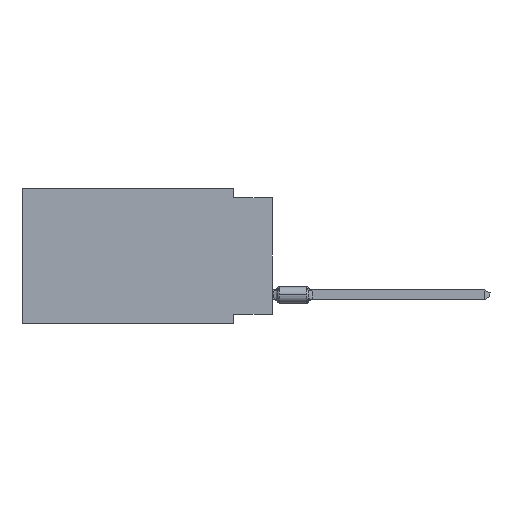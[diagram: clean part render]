
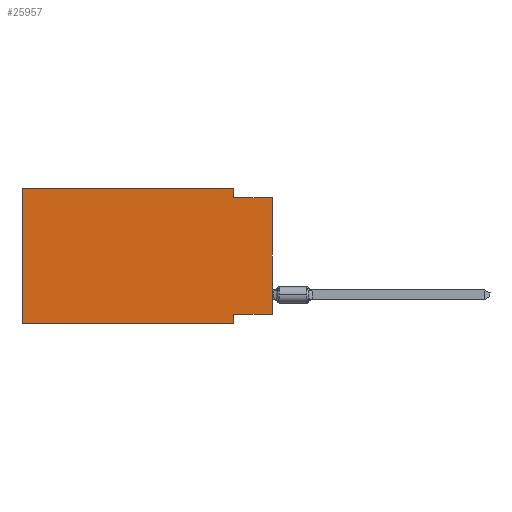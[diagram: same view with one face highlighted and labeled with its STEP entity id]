
A CAD part, left-side view. The second image highlights one B-rep face of the part: STEP entity #25957.
In plain terms, the highlighted planar face has unit normal (-1, 0, 0).
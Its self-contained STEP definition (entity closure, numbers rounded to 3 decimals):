
#1000 = DIRECTION ( 'NONE',  ( 0., 0., -1. ) ) ;
#1112 = DIRECTION ( 'NONE',  ( 0., 0., -1. ) ) ;
#1555 = ORIENTED_EDGE ( 'NONE', *, *, #27193, .F. ) ;
#2765 = ORIENTED_EDGE ( 'NONE', *, *, #39195, .F. ) ;
#4514 = CARTESIAN_POINT ( 'NONE',  ( 0., 2.54, 0. ) ) ;
#4989 = EDGE_CURVE ( 'NONE', #33740, #26155, #41452, .T. ) ;
#5279 = AXIS2_PLACEMENT_3D ( 'NONE', #33440, #35003, #1112 ) ;
#5985 = PLANE ( 'NONE',  #5279 ) ;
#6275 = LINE ( 'NONE', #20686, #9706 ) ;
#6925 = ORIENTED_EDGE ( 'NONE', *, *, #11265, .F. ) ;
#7074 = LINE ( 'NONE', #42701, #24734 ) ;
#8180 = FACE_OUTER_BOUND ( 'NONE', #15157, .T. ) ;
#8844 = LINE ( 'NONE', #19970, #28362 ) ;
#9148 = LINE ( 'NONE', #15763, #44595 ) ;
#9351 = ORIENTED_EDGE ( 'NONE', *, *, #15860, .F. ) ;
#9706 = VECTOR ( 'NONE', #35748, 1000. ) ;
#9810 = LINE ( 'NONE', #10257, #33088 ) ;
#10257 = CARTESIAN_POINT ( 'NONE',  ( 0., 16.383, 0. ) ) ;
#10415 = CARTESIAN_POINT ( 'NONE',  ( 0., 0., -8.255 ) ) ;
#11008 = CARTESIAN_POINT ( 'NONE',  ( 0., 16.383, 0. ) ) ;
#11265 = EDGE_CURVE ( 'NONE', #23553, #26155, #7074, .T. ) ;
#13021 = LINE ( 'NONE', #16814, #21232 ) ;
#13597 = CARTESIAN_POINT ( 'NONE',  ( 0., 0., 0. ) ) ;
#13998 = CARTESIAN_POINT ( 'NONE',  ( 0., 0., -0.635 ) ) ;
#15157 = EDGE_LOOP ( 'NONE', ( #38089, #6925, #9351, #1555, #43843, #21561, #2765, #21876 ) ) ;
#15763 = CARTESIAN_POINT ( 'NONE',  ( 0., 16.383, 0. ) ) ;
#15860 = EDGE_CURVE ( 'NONE', #34792, #23553, #33320, .T. ) ;
#16075 = CARTESIAN_POINT ( 'NONE',  ( 0., 2.54, -8.255 ) ) ;
#16814 = CARTESIAN_POINT ( 'NONE',  ( 0., 0., -8.255 ) ) ;
#19796 = DIRECTION ( 'NONE',  ( 0., -1., 0. ) ) ;
#19970 = CARTESIAN_POINT ( 'NONE',  ( 0., 16.383, -8.89 ) ) ;
#20492 = VERTEX_POINT ( 'NONE', #16075 ) ;
#20686 = CARTESIAN_POINT ( 'NONE',  ( 0., 2.54, -8.89 ) ) ;
#21076 = VECTOR ( 'NONE', #1000, 1000. ) ;
#21232 = VECTOR ( 'NONE', #38712, 1000. ) ;
#21561 = ORIENTED_EDGE ( 'NONE', *, *, #43914, .T. ) ;
#21876 = ORIENTED_EDGE ( 'NONE', *, *, #28725, .F. ) ;
#23553 = VERTEX_POINT ( 'NONE', #26669 ) ;
#24734 = VECTOR ( 'NONE', #35388, 1000. ) ;
#25062 = VECTOR ( 'NONE', #27729, 1000. ) ;
#25734 = VERTEX_POINT ( 'NONE', #45717 ) ;
#25957 = ADVANCED_FACE ( 'NONE', ( #8180 ), #5985, .F. ) ;
#26155 = VERTEX_POINT ( 'NONE', #13998 ) ;
#26669 = CARTESIAN_POINT ( 'NONE',  ( 0., 2.54, -0.635 ) ) ;
#26938 = VERTEX_POINT ( 'NONE', #46213 ) ;
#27193 = EDGE_CURVE ( 'NONE', #38830, #34792, #9148, .T. ) ;
#27729 = DIRECTION ( 'NONE',  ( 0., 0., 1. ) ) ;
#28362 = VECTOR ( 'NONE', #44728, 1000. ) ;
#28725 = EDGE_CURVE ( 'NONE', #33740, #20492, #13021, .T. ) ;
#33088 = VECTOR ( 'NONE', #42838, 1000. ) ;
#33320 = LINE ( 'NONE', #4514, #21076 ) ;
#33440 = CARTESIAN_POINT ( 'NONE',  ( 0., 16.383, 0. ) ) ;
#33740 = VERTEX_POINT ( 'NONE', #10415 ) ;
#34792 = VERTEX_POINT ( 'NONE', #34869 ) ;
#34869 = CARTESIAN_POINT ( 'NONE',  ( 0., 2.54, 0. ) ) ;
#35003 = DIRECTION ( 'NONE',  ( 1., 0., 0. ) ) ;
#35388 = DIRECTION ( 'NONE',  ( 0., -1., 0. ) ) ;
#35517 = EDGE_CURVE ( 'NONE', #26938, #38830, #9810, .T. ) ;
#35748 = DIRECTION ( 'NONE',  ( 0., 0., -1. ) ) ;
#38089 = ORIENTED_EDGE ( 'NONE', *, *, #4989, .T. ) ;
#38712 = DIRECTION ( 'NONE',  ( 0., 1., 0. ) ) ;
#38830 = VERTEX_POINT ( 'NONE', #11008 ) ;
#39195 = EDGE_CURVE ( 'NONE', #20492, #25734, #6275, .T. ) ;
#41452 = LINE ( 'NONE', #13597, #25062 ) ;
#42701 = CARTESIAN_POINT ( 'NONE',  ( 0., 0., -0.635 ) ) ;
#42838 = DIRECTION ( 'NONE',  ( 0., 0., 1. ) ) ;
#43843 = ORIENTED_EDGE ( 'NONE', *, *, #35517, .F. ) ;
#43914 = EDGE_CURVE ( 'NONE', #26938, #25734, #8844, .T. ) ;
#44595 = VECTOR ( 'NONE', #19796, 1000. ) ;
#44728 = DIRECTION ( 'NONE',  ( 0., -1., 0. ) ) ;
#45717 = CARTESIAN_POINT ( 'NONE',  ( 0., 2.54, -8.89 ) ) ;
#46213 = CARTESIAN_POINT ( 'NONE',  ( 0., 16.383, -8.89 ) ) ;
